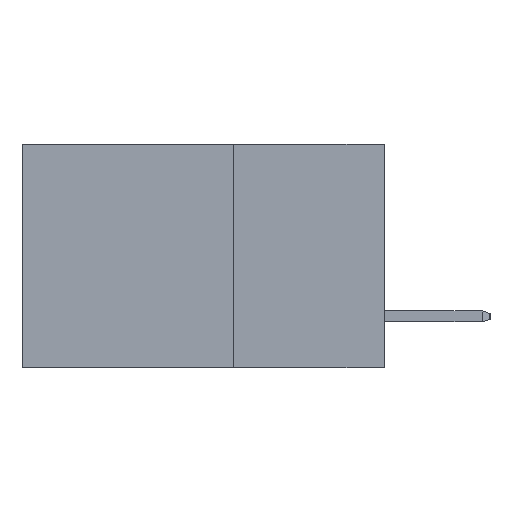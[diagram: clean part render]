
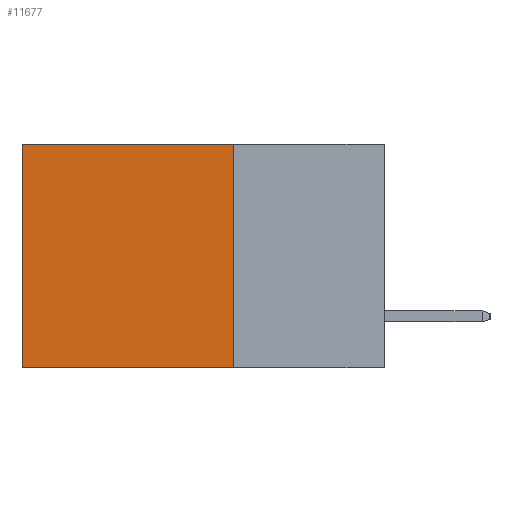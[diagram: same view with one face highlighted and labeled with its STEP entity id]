
A CAD part, left-side view. The second image highlights one B-rep face of the part: STEP entity #11677.
In plain terms, the highlighted planar face has unit normal (-1, 0, 0).
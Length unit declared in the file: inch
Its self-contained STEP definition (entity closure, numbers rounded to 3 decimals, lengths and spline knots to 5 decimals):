
#772 = VERTEX_POINT ( 'NONE', #14829 ) ;
#812 = LINE ( 'NONE', #10410, #10468 ) ;
#1881 = CARTESIAN_POINT ( 'NONE',  ( 0.2615, 0.25, -0.37 ) ) ;
#1944 = LINE ( 'NONE', #14569, #15581 ) ;
#2373 = EDGE_CURVE ( 'NONE', #772, #6816, #1944, .T. ) ;
#2838 = ORIENTED_EDGE ( 'NONE', *, *, #2373, .F. ) ;
#3229 = VECTOR ( 'NONE', #3709, 39.37008 ) ;
#3248 = EDGE_LOOP ( 'NONE', ( #22330, #8018, #2838, #14008 ) ) ;
#3709 = DIRECTION ( 'NONE',  ( 0., 1., 0. ) ) ;
#6572 = EDGE_CURVE ( 'NONE', #772, #19741, #14726, .T. ) ;
#6816 = VERTEX_POINT ( 'NONE', #16733 ) ;
#8018 = ORIENTED_EDGE ( 'NONE', *, *, #20571, .F. ) ;
#9302 = AXIS2_PLACEMENT_3D ( 'NONE', #19119, #16889, #16518 ) ;
#9924 = CARTESIAN_POINT ( 'NONE',  ( 0.2615, 0.6, 0. ) ) ;
#10392 = DIRECTION ( 'NONE',  ( 0., 0., -1. ) ) ;
#10410 = CARTESIAN_POINT ( 'NONE',  ( 0.2615, 0.6, -0.37 ) ) ;
#10468 = VECTOR ( 'NONE', #10392, 39.37008 ) ;
#11677 = ADVANCED_FACE ( 'NONE', ( #21330 ), #18668, .F. ) ;
#12741 = LINE ( 'NONE', #1881, #3229 ) ;
#14008 = ORIENTED_EDGE ( 'NONE', *, *, #6572, .T. ) ;
#14339 = DIRECTION ( 'NONE',  ( 0., 0., -1. ) ) ;
#14569 = CARTESIAN_POINT ( 'NONE',  ( 0.2615, 0.25, -0.37 ) ) ;
#14726 = LINE ( 'NONE', #21226, #22512 ) ;
#14779 = VERTEX_POINT ( 'NONE', #19606 ) ;
#14829 = CARTESIAN_POINT ( 'NONE',  ( 0.2615, 0.25, 0. ) ) ;
#15581 = VECTOR ( 'NONE', #14339, 39.37008 ) ;
#16518 = DIRECTION ( 'NONE',  ( 0., 0., -1. ) ) ;
#16562 = EDGE_CURVE ( 'NONE', #19741, #14779, #812, .T. ) ;
#16733 = CARTESIAN_POINT ( 'NONE',  ( 0.2615, 0.25, -0.37 ) ) ;
#16889 = DIRECTION ( 'NONE',  ( 1., 0., 0. ) ) ;
#18668 = PLANE ( 'NONE',  #9302 ) ;
#19119 = CARTESIAN_POINT ( 'NONE',  ( 0.2615, 0.25, -0.37 ) ) ;
#19606 = CARTESIAN_POINT ( 'NONE',  ( 0.2615, 0.6, -0.37 ) ) ;
#19741 = VERTEX_POINT ( 'NONE', #9924 ) ;
#20571 = EDGE_CURVE ( 'NONE', #6816, #14779, #12741, .T. ) ;
#21226 = CARTESIAN_POINT ( 'NONE',  ( 0.2615, 0.25, 0. ) ) ;
#21330 = FACE_OUTER_BOUND ( 'NONE', #3248, .T. ) ;
#21495 = DIRECTION ( 'NONE',  ( 0., 1., 0. ) ) ;
#22330 = ORIENTED_EDGE ( 'NONE', *, *, #16562, .T. ) ;
#22512 = VECTOR ( 'NONE', #21495, 39.37008 ) ;
